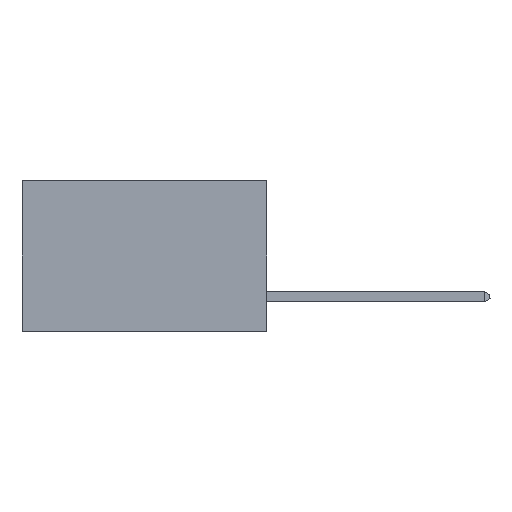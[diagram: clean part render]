
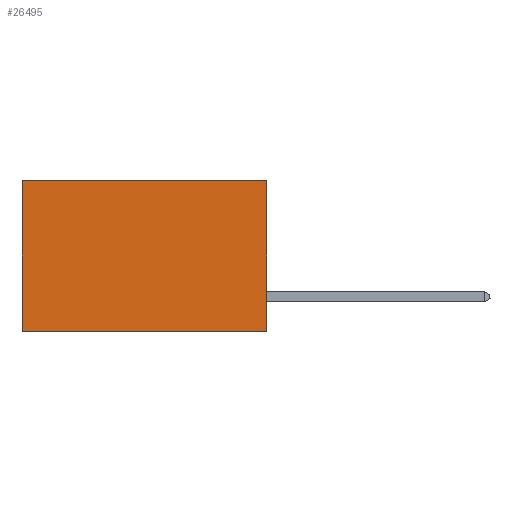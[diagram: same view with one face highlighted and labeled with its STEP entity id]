
A CAD part, left-side view. The second image highlights one B-rep face of the part: STEP entity #26495.
In plain terms, the highlighted planar face has unit normal (-1, 0, 0).
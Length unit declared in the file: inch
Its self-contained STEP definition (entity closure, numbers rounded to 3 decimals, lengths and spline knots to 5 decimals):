
#862 = VECTOR ( 'NONE', #9531, 39.37008 ) ;
#1238 = ORIENTED_EDGE ( 'NONE', *, *, #13974, .F. ) ;
#2088 = VECTOR ( 'NONE', #15063, 39.37008 ) ;
#2253 = ORIENTED_EDGE ( 'NONE', *, *, #3344, .F. ) ;
#3344 = EDGE_CURVE ( 'NONE', #19440, #4107, #28183, .T. ) ;
#4107 = VERTEX_POINT ( 'NONE', #22624 ) ;
#5974 = DIRECTION ( 'NONE',  ( 0., 0., -1. ) ) ;
#9531 = DIRECTION ( 'NONE',  ( 0., 1., 0. ) ) ;
#9681 = EDGE_LOOP ( 'NONE', ( #10038, #1238, #2253, #13836 ) ) ;
#10038 = ORIENTED_EDGE ( 'NONE', *, *, #27217, .T. ) ;
#10088 = DIRECTION ( 'NONE',  ( 1., 0., 0. ) ) ;
#10093 = CARTESIAN_POINT ( 'NONE',  ( 0.2875, 0., -0.37 ) ) ;
#10596 = CARTESIAN_POINT ( 'NONE',  ( 0.2875, 0., 0. ) ) ;
#10856 = CARTESIAN_POINT ( 'NONE',  ( 0.2875, 0.6, 0. ) ) ;
#11053 = DIRECTION ( 'NONE',  ( 0., 0., -1. ) ) ;
#12416 = LINE ( 'NONE', #10093, #20788 ) ;
#12439 = PLANE ( 'NONE',  #24294 ) ;
#13836 = ORIENTED_EDGE ( 'NONE', *, *, #14547, .T. ) ;
#13974 = EDGE_CURVE ( 'NONE', #4107, #28842, #12416, .T. ) ;
#14536 = CARTESIAN_POINT ( 'NONE',  ( 0.2875, 0.6, -0.37 ) ) ;
#14547 = EDGE_CURVE ( 'NONE', #19440, #14985, #21802, .T. ) ;
#14665 = CARTESIAN_POINT ( 'NONE',  ( 0.2875, 0., 0. ) ) ;
#14985 = VERTEX_POINT ( 'NONE', #22002 ) ;
#15063 = DIRECTION ( 'NONE',  ( 0., 0., -1. ) ) ;
#19440 = VERTEX_POINT ( 'NONE', #21722 ) ;
#19686 = FACE_OUTER_BOUND ( 'NONE', #9681, .T. ) ;
#19998 = VECTOR ( 'NONE', #11053, 39.37008 ) ;
#20788 = VECTOR ( 'NONE', #23071, 39.37008 ) ;
#21722 = CARTESIAN_POINT ( 'NONE',  ( 0.2875, 0., 0. ) ) ;
#21802 = LINE ( 'NONE', #25200, #862 ) ;
#22002 = CARTESIAN_POINT ( 'NONE',  ( 0.2875, 0.6, 0. ) ) ;
#22624 = CARTESIAN_POINT ( 'NONE',  ( 0.2875, 0., -0.37 ) ) ;
#23071 = DIRECTION ( 'NONE',  ( 0., 1., 0. ) ) ;
#24294 = AXIS2_PLACEMENT_3D ( 'NONE', #14665, #10088, #5974 ) ;
#25200 = CARTESIAN_POINT ( 'NONE',  ( 0.2875, 0., 0. ) ) ;
#26495 = ADVANCED_FACE ( 'NONE', ( #19686 ), #12439, .F. ) ;
#27217 = EDGE_CURVE ( 'NONE', #14985, #28842, #27987, .T. ) ;
#27987 = LINE ( 'NONE', #10856, #19998 ) ;
#28183 = LINE ( 'NONE', #10596, #2088 ) ;
#28842 = VERTEX_POINT ( 'NONE', #14536 ) ;
